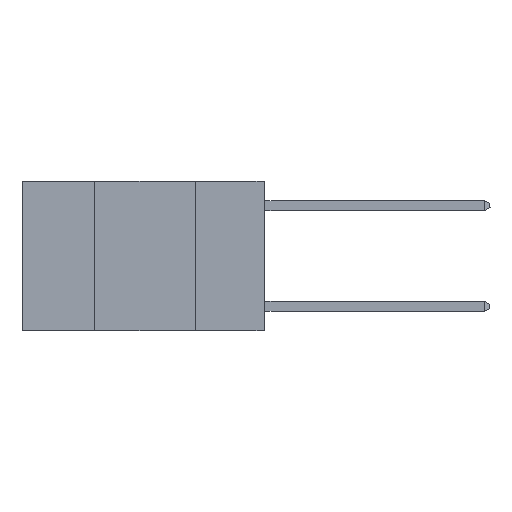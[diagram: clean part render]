
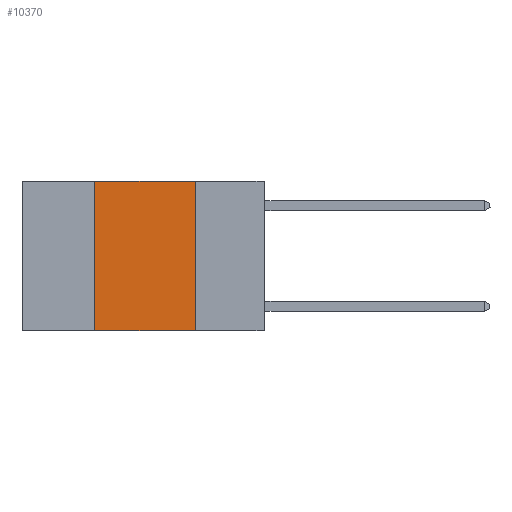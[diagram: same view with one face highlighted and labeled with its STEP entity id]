
A CAD part, left-side view. The second image highlights one B-rep face of the part: STEP entity #10370.
In plain terms, the highlighted planar face has unit normal (-1, 0, 0).
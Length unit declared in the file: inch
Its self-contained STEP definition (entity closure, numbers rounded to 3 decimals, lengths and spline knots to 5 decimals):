
#223 = ORIENTED_EDGE ( 'NONE', *, *, #2438, .F. ) ;
#749 = LINE ( 'NONE', #12982, #7415 ) ;
#1454 = CARTESIAN_POINT ( 'NONE',  ( 0., 0.6, 0. ) ) ;
#2392 = CARTESIAN_POINT ( 'NONE',  ( 0., 0.6, 0. ) ) ;
#2438 = EDGE_CURVE ( 'NONE', #11357, #16409, #13035, .T. ) ;
#2505 = DIRECTION ( 'NONE',  ( 0., -1., 0. ) ) ;
#2810 = DIRECTION ( 'NONE',  ( 1., 0., 0. ) ) ;
#3346 = LINE ( 'NONE', #7499, #16734 ) ;
#3497 = FACE_OUTER_BOUND ( 'NONE', #6925, .T. ) ;
#3607 = EDGE_CURVE ( 'NONE', #5740, #11357, #3346, .T. ) ;
#3633 = CARTESIAN_POINT ( 'NONE',  ( 0., 0.17, 0. ) ) ;
#3677 = DIRECTION ( 'NONE',  ( 0., -1., 0. ) ) ;
#3711 = ORIENTED_EDGE ( 'NONE', *, *, #3607, .F. ) ;
#4501 = EDGE_CURVE ( 'NONE', #16409, #8072, #11590, .T. ) ;
#4967 = CARTESIAN_POINT ( 'NONE',  ( 0., 0.17, 0. ) ) ;
#5026 = DIRECTION ( 'NONE',  ( 0., 0., -1. ) ) ;
#5740 = VERTEX_POINT ( 'NONE', #15047 ) ;
#6644 = EDGE_CURVE ( 'NONE', #5740, #8072, #749, .T. ) ;
#6856 = ORIENTED_EDGE ( 'NONE', *, *, #4501, .F. ) ;
#6925 = EDGE_LOOP ( 'NONE', ( #6856, #223, #3711, #7278 ) ) ;
#7278 = ORIENTED_EDGE ( 'NONE', *, *, #6644, .T. ) ;
#7289 = CARTESIAN_POINT ( 'NONE',  ( 0., 0.17, -0.37 ) ) ;
#7415 = VECTOR ( 'NONE', #2505, 39.37008 ) ;
#7499 = CARTESIAN_POINT ( 'NONE',  ( 0., 0.42, 0. ) ) ;
#8072 = VERTEX_POINT ( 'NONE', #7289 ) ;
#10370 = ADVANCED_FACE ( 'NONE', ( #3497 ), #10735, .F. ) ;
#10735 = PLANE ( 'NONE',  #13437 ) ;
#10794 = VECTOR ( 'NONE', #5026, 39.37008 ) ;
#11357 = VERTEX_POINT ( 'NONE', #11460 ) ;
#11460 = CARTESIAN_POINT ( 'NONE',  ( 0., 0.42, 0. ) ) ;
#11590 = LINE ( 'NONE', #4967, #10794 ) ;
#12026 = DIRECTION ( 'NONE',  ( 0., 0., -1. ) ) ;
#12733 = DIRECTION ( 'NONE',  ( 0., 0., 1. ) ) ;
#12982 = CARTESIAN_POINT ( 'NONE',  ( 0., 0.6, -0.37 ) ) ;
#13035 = LINE ( 'NONE', #2392, #15990 ) ;
#13437 = AXIS2_PLACEMENT_3D ( 'NONE', #1454, #2810, #12026 ) ;
#15047 = CARTESIAN_POINT ( 'NONE',  ( 0., 0.42, -0.37 ) ) ;
#15990 = VECTOR ( 'NONE', #3677, 39.37008 ) ;
#16409 = VERTEX_POINT ( 'NONE', #3633 ) ;
#16734 = VECTOR ( 'NONE', #12733, 39.37008 ) ;
